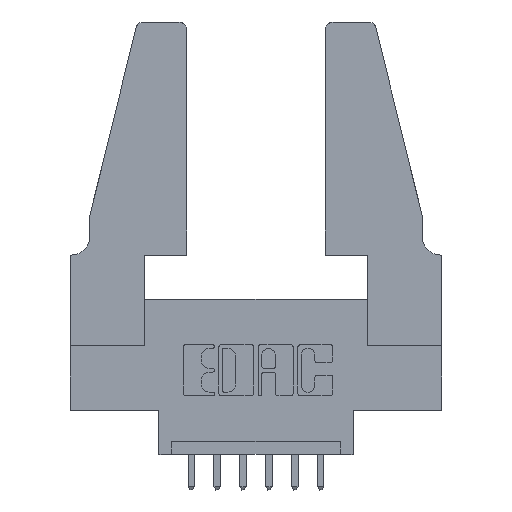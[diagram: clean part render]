
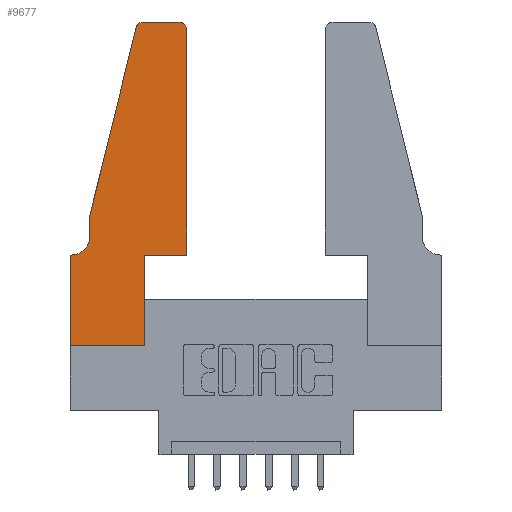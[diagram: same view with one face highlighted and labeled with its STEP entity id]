
A CAD part, top view. The second image highlights one B-rep face of the part: STEP entity #9677.
In plain terms, the highlighted planar face has unit normal (0, 0, 1).
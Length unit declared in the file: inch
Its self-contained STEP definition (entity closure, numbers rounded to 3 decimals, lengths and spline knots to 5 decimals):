
#49 = DIRECTION ( 'NONE',  ( -1., 0., 0. ) ) ;
#151 = LINE ( 'NONE', #5420, #851 ) ;
#157 = VERTEX_POINT ( 'NONE', #10002 ) ;
#162 = VECTOR ( 'NONE', #2215, 39.37008 ) ;
#223 = CIRCLE ( 'NONE', #9490, 0.07 ) ;
#277 = CIRCLE ( 'NONE', #4209, 0.03 ) ;
#312 = CARTESIAN_POINT ( 'NONE',  ( 0.0055, 0.35, 0.37 ) ) ;
#383 = LINE ( 'NONE', #11328, #5010 ) ;
#762 = LINE ( 'NONE', #3346, #1043 ) ;
#800 = DIRECTION ( 'NONE',  ( 0., 1., 0. ) ) ;
#851 = VECTOR ( 'NONE', #49, 39.37008 ) ;
#945 = VERTEX_POINT ( 'NONE', #6001 ) ;
#979 = VECTOR ( 'NONE', #7239, 39.37008 ) ;
#1043 = VECTOR ( 'NONE', #7739, 39.37008 ) ;
#1188 = ORIENTED_EDGE ( 'NONE', *, *, #10838, .T. ) ;
#1471 = CARTESIAN_POINT ( 'NONE',  ( 0.0755, 0.42, 0.37 ) ) ;
#1579 = CARTESIAN_POINT ( 'NONE',  ( 0.0755, 0.5, 0.37 ) ) ;
#1622 = ORIENTED_EDGE ( 'NONE', *, *, #4318, .T. ) ;
#1942 = CARTESIAN_POINT ( 'NONE',  ( 0.4205, 1.25, 0.37 ) ) ;
#2021 = EDGE_CURVE ( 'NONE', #10201, #7627, #6616, .T. ) ;
#2061 = CARTESIAN_POINT ( 'NONE',  ( 0.2865, 0., 0.37 ) ) ;
#2167 = CARTESIAN_POINT ( 'NONE',  ( 0.284, 1.22, 0.37 ) ) ;
#2202 = EDGE_CURVE ( 'NONE', #11064, #7746, #151, .T. ) ;
#2215 = DIRECTION ( 'NONE',  ( 0., -1., 0. ) ) ;
#2261 = EDGE_CURVE ( 'NONE', #7746, #7352, #4503, .T. ) ;
#2475 = CARTESIAN_POINT ( 'NONE',  ( 0.0055, 0.42, 0.37 ) ) ;
#2582 = EDGE_LOOP ( 'NONE', ( #1622, #5704, #4600, #5049, #9263, #8113, #3626, #1188, #8220, #5141, #4531, #5373 ) ) ;
#2592 = CARTESIAN_POINT ( 'NONE',  ( 0.4505, 0.35, 0.37 ) ) ;
#2851 = VECTOR ( 'NONE', #11157, 39.37008 ) ;
#3120 = DIRECTION ( 'NONE',  ( 1., 0., 0. ) ) ;
#3214 = CARTESIAN_POINT ( 'NONE',  ( 0.0755, 0.5, 0.37 ) ) ;
#3273 = LINE ( 'NONE', #3214, #162 ) ;
#3346 = CARTESIAN_POINT ( 'NONE',  ( 0., 0., 0.37 ) ) ;
#3413 = DIRECTION ( 'NONE',  ( -0.239, -0.971, 0. ) ) ;
#3450 = VERTEX_POINT ( 'NONE', #1942 ) ;
#3626 = ORIENTED_EDGE ( 'NONE', *, *, #2261, .T. ) ;
#3769 = PLANE ( 'NONE',  #4471 ) ;
#3821 = VECTOR ( 'NONE', #800, 39.37008 ) ;
#3884 = EDGE_CURVE ( 'NONE', #7627, #6610, #383, .T. ) ;
#4209 = AXIS2_PLACEMENT_3D ( 'NONE', #2167, #5748, #8473 ) ;
#4261 = DIRECTION ( 'NONE',  ( 0., 1., 0. ) ) ;
#4318 = EDGE_CURVE ( 'NONE', #3450, #157, #7132, .T. ) ;
#4414 = CARTESIAN_POINT ( 'NONE',  ( 0.2865, 0.35, 0.37 ) ) ;
#4471 = AXIS2_PLACEMENT_3D ( 'NONE', #10951, #9917, #7220 ) ;
#4503 = LINE ( 'NONE', #8124, #979 ) ;
#4531 = ORIENTED_EDGE ( 'NONE', *, *, #3884, .T. ) ;
#4600 = ORIENTED_EDGE ( 'NONE', *, *, #5933, .T. ) ;
#4648 = AXIS2_PLACEMENT_3D ( 'NONE', #5811, #11207, #3120 ) ;
#4858 = VECTOR ( 'NONE', #6663, 39.37008 ) ;
#5010 = VECTOR ( 'NONE', #4261, 39.37008 ) ;
#5049 = ORIENTED_EDGE ( 'NONE', *, *, #7223, .T. ) ;
#5069 = VERTEX_POINT ( 'NONE', #7155 ) ;
#5141 = ORIENTED_EDGE ( 'NONE', *, *, #2021, .T. ) ;
#5152 = DIRECTION ( 'NONE',  ( 0., 0., -1. ) ) ;
#5213 = EDGE_CURVE ( 'NONE', #11619, #11064, #223, .T. ) ;
#5373 = ORIENTED_EDGE ( 'NONE', *, *, #5523, .T. ) ;
#5420 = CARTESIAN_POINT ( 'NONE',  ( 0.0755, 0.35, 0.37 ) ) ;
#5523 = EDGE_CURVE ( 'NONE', #6610, #3450, #9791, .T. ) ;
#5586 = CARTESIAN_POINT ( 'NONE',  ( 0.4505, 1.22, 0.37 ) ) ;
#5704 = ORIENTED_EDGE ( 'NONE', *, *, #8562, .T. ) ;
#5748 = DIRECTION ( 'NONE',  ( 0., 0., 1. ) ) ;
#5811 = CARTESIAN_POINT ( 'NONE',  ( 0.4205, 1.22, 0.37 ) ) ;
#5933 = EDGE_CURVE ( 'NONE', #945, #5069, #10924, .T. ) ;
#6001 = CARTESIAN_POINT ( 'NONE',  ( 0.25487, 1.22718, 0.37 ) ) ;
#6126 = FACE_OUTER_BOUND ( 'NONE', #2582, .T. ) ;
#6610 = VERTEX_POINT ( 'NONE', #5586 ) ;
#6616 = LINE ( 'NONE', #2592, #2851 ) ;
#6663 = DIRECTION ( 'NONE',  ( -1., 0., 0. ) ) ;
#7132 = LINE ( 'NONE', #8401, #4858 ) ;
#7155 = CARTESIAN_POINT ( 'NONE',  ( 0.0755, 0.5, 0.37 ) ) ;
#7220 = DIRECTION ( 'NONE',  ( 1., 0., 0. ) ) ;
#7223 = EDGE_CURVE ( 'NONE', #5069, #11619, #3273, .T. ) ;
#7239 = DIRECTION ( 'NONE',  ( 0., -1., 0. ) ) ;
#7352 = VERTEX_POINT ( 'NONE', #10814 ) ;
#7512 = CARTESIAN_POINT ( 'NONE',  ( 0., 0.35, 0.37 ) ) ;
#7571 = EDGE_CURVE ( 'NONE', #10875, #10201, #9056, .T. ) ;
#7627 = VERTEX_POINT ( 'NONE', #9783 ) ;
#7739 = DIRECTION ( 'NONE',  ( 1., 0., 0. ) ) ;
#7746 = VERTEX_POINT ( 'NONE', #7512 ) ;
#7816 = VECTOR ( 'NONE', #3413, 39.37008 ) ;
#7869 = CARTESIAN_POINT ( 'NONE',  ( 0.2865, 0.35, 0.37 ) ) ;
#8113 = ORIENTED_EDGE ( 'NONE', *, *, #2202, .T. ) ;
#8124 = CARTESIAN_POINT ( 'NONE',  ( 0., 0., 0.37 ) ) ;
#8220 = ORIENTED_EDGE ( 'NONE', *, *, #7571, .T. ) ;
#8401 = CARTESIAN_POINT ( 'NONE',  ( 0.2605, 1.25, 0.37 ) ) ;
#8473 = DIRECTION ( 'NONE',  ( 1., 0., 0. ) ) ;
#8562 = EDGE_CURVE ( 'NONE', #157, #945, #277, .T. ) ;
#9056 = LINE ( 'NONE', #4414, #3821 ) ;
#9263 = ORIENTED_EDGE ( 'NONE', *, *, #5213, .T. ) ;
#9490 = AXIS2_PLACEMENT_3D ( 'NONE', #2475, #5152, #10533 ) ;
#9677 = ADVANCED_FACE ( 'NONE', ( #6126 ), #3769, .T. ) ;
#9783 = CARTESIAN_POINT ( 'NONE',  ( 0.4505, 0.35, 0.37 ) ) ;
#9791 = CIRCLE ( 'NONE', #4648, 0.03 ) ;
#9917 = DIRECTION ( 'NONE',  ( 0., 0., 1. ) ) ;
#10002 = CARTESIAN_POINT ( 'NONE',  ( 0.284, 1.25, 0.37 ) ) ;
#10201 = VERTEX_POINT ( 'NONE', #7869 ) ;
#10533 = DIRECTION ( 'NONE',  ( -1., 0., 0. ) ) ;
#10814 = CARTESIAN_POINT ( 'NONE',  ( 0., 0., 0.37 ) ) ;
#10838 = EDGE_CURVE ( 'NONE', #7352, #10875, #762, .T. ) ;
#10875 = VERTEX_POINT ( 'NONE', #2061 ) ;
#10924 = LINE ( 'NONE', #1579, #7816 ) ;
#10951 = CARTESIAN_POINT ( 'NONE',  ( 0., 0.35, 0.37 ) ) ;
#11064 = VERTEX_POINT ( 'NONE', #312 ) ;
#11157 = DIRECTION ( 'NONE',  ( 1., 0., 0. ) ) ;
#11207 = DIRECTION ( 'NONE',  ( 0., 0., 1. ) ) ;
#11328 = CARTESIAN_POINT ( 'NONE',  ( 0.4505, 0.35, 0.37 ) ) ;
#11619 = VERTEX_POINT ( 'NONE', #1471 ) ;
